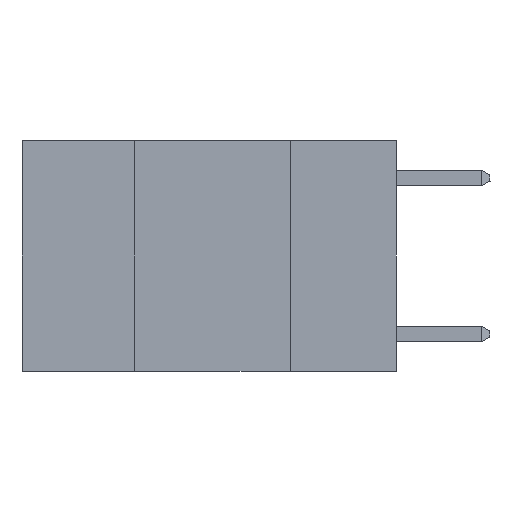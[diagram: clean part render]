
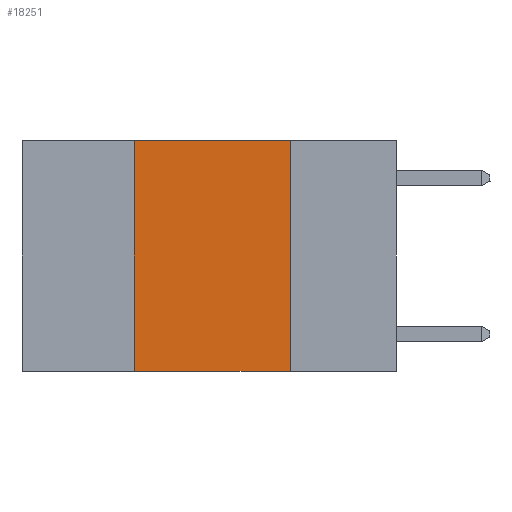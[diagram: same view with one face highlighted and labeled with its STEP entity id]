
A CAD part, left-side view. The second image highlights one B-rep face of the part: STEP entity #18251.
In plain terms, the highlighted planar face has unit normal (-1, 0, 0).
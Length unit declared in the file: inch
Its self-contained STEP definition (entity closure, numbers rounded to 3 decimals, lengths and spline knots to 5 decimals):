
#811 = VECTOR ( 'NONE', #23034, 39.37008 ) ;
#2629 = VERTEX_POINT ( 'NONE', #9791 ) ;
#3830 = EDGE_CURVE ( 'NONE', #6144, #2629, #13698, .T. ) ;
#5999 = PLANE ( 'NONE',  #8071 ) ;
#6144 = VERTEX_POINT ( 'NONE', #8423 ) ;
#6721 = EDGE_CURVE ( 'NONE', #6144, #6997, #11913, .T. ) ;
#6997 = VERTEX_POINT ( 'NONE', #12730 ) ;
#7490 = EDGE_CURVE ( 'NONE', #16228, #6997, #19559, .T. ) ;
#8071 = AXIS2_PLACEMENT_3D ( 'NONE', #9692, #22304, #11491 ) ;
#8423 = CARTESIAN_POINT ( 'NONE',  ( 0., 0.42, -0.37 ) ) ;
#8629 = ORIENTED_EDGE ( 'NONE', *, *, #7490, .F. ) ;
#8845 = ORIENTED_EDGE ( 'NONE', *, *, #19162, .F. ) ;
#9386 = CARTESIAN_POINT ( 'NONE',  ( 0., 0.6, 0. ) ) ;
#9560 = ORIENTED_EDGE ( 'NONE', *, *, #3830, .F. ) ;
#9627 = ORIENTED_EDGE ( 'NONE', *, *, #6721, .T. ) ;
#9692 = CARTESIAN_POINT ( 'NONE',  ( 0., 0.6, 0. ) ) ;
#9791 = CARTESIAN_POINT ( 'NONE',  ( 0., 0.42, 0. ) ) ;
#10371 = LINE ( 'NONE', #9386, #15173 ) ;
#11491 = DIRECTION ( 'NONE',  ( 0., 0., -1. ) ) ;
#11913 = LINE ( 'NONE', #22905, #17334 ) ;
#12108 = DIRECTION ( 'NONE',  ( 0., -1., 0. ) ) ;
#12616 = CARTESIAN_POINT ( 'NONE',  ( 0., 0.42, 0. ) ) ;
#12730 = CARTESIAN_POINT ( 'NONE',  ( 0., 0.17, -0.37 ) ) ;
#13698 = LINE ( 'NONE', #12616, #22725 ) ;
#14363 = DIRECTION ( 'NONE',  ( 0., 0., 1. ) ) ;
#14396 = EDGE_LOOP ( 'NONE', ( #8629, #8845, #9560, #9627 ) ) ;
#15173 = VECTOR ( 'NONE', #22014, 39.37008 ) ;
#16228 = VERTEX_POINT ( 'NONE', #18958 ) ;
#16357 = FACE_OUTER_BOUND ( 'NONE', #14396, .T. ) ;
#17334 = VECTOR ( 'NONE', #12108, 39.37008 ) ;
#18251 = ADVANCED_FACE ( 'NONE', ( #16357 ), #5999, .F. ) ;
#18958 = CARTESIAN_POINT ( 'NONE',  ( 0., 0.17, 0. ) ) ;
#19162 = EDGE_CURVE ( 'NONE', #2629, #16228, #10371, .T. ) ;
#19559 = LINE ( 'NONE', #21254, #811 ) ;
#21254 = CARTESIAN_POINT ( 'NONE',  ( 0., 0.17, 0. ) ) ;
#22014 = DIRECTION ( 'NONE',  ( 0., -1., 0. ) ) ;
#22304 = DIRECTION ( 'NONE',  ( 1., 0., 0. ) ) ;
#22725 = VECTOR ( 'NONE', #14363, 39.37008 ) ;
#22905 = CARTESIAN_POINT ( 'NONE',  ( 0., 0.6, -0.37 ) ) ;
#23034 = DIRECTION ( 'NONE',  ( 0., 0., -1. ) ) ;
